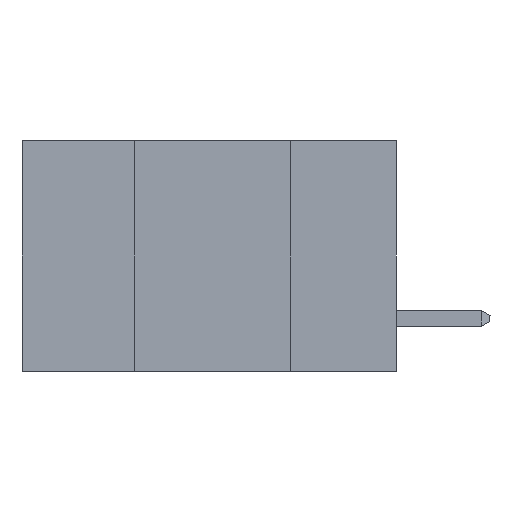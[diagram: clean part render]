
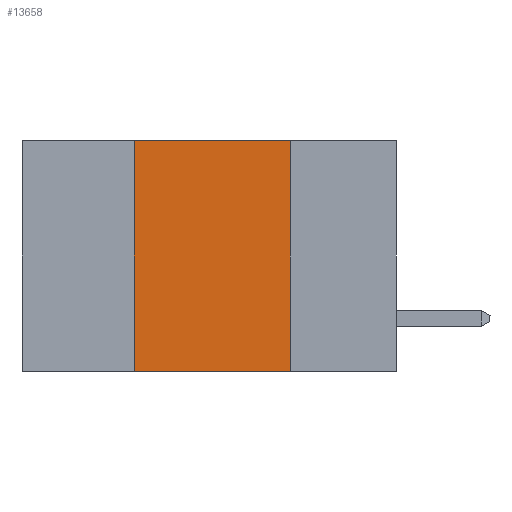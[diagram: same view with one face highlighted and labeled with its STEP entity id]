
A CAD part, left-side view. The second image highlights one B-rep face of the part: STEP entity #13658.
In plain terms, the highlighted planar face has unit normal (-1, 0, 0).
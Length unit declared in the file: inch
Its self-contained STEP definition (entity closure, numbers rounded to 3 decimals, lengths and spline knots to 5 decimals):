
#482 = EDGE_CURVE ( 'NONE', #15185, #2514, #15373, .T. ) ;
#598 = VERTEX_POINT ( 'NONE', #4691 ) ;
#778 = CARTESIAN_POINT ( 'NONE',  ( 0., 0.42, -0.37 ) ) ;
#888 = CARTESIAN_POINT ( 'NONE',  ( 0., 0.6, 0. ) ) ;
#2514 = VERTEX_POINT ( 'NONE', #10790 ) ;
#3417 = EDGE_LOOP ( 'NONE', ( #11002, #4985, #3614, #9863 ) ) ;
#3520 = DIRECTION ( 'NONE',  ( 0., 0., -1. ) ) ;
#3614 = ORIENTED_EDGE ( 'NONE', *, *, #12351, .F. ) ;
#3699 = VECTOR ( 'NONE', #4540, 39.37008 ) ;
#3708 = LINE ( 'NONE', #6241, #10955 ) ;
#3782 = DIRECTION ( 'NONE',  ( 0., 0., -1. ) ) ;
#4019 = VERTEX_POINT ( 'NONE', #778 ) ;
#4316 = LINE ( 'NONE', #14029, #6190 ) ;
#4540 = DIRECTION ( 'NONE',  ( 0., -1., 0. ) ) ;
#4691 = CARTESIAN_POINT ( 'NONE',  ( 0., 0.17, -0.37 ) ) ;
#4985 = ORIENTED_EDGE ( 'NONE', *, *, #482, .F. ) ;
#6190 = VECTOR ( 'NONE', #7683, 39.37008 ) ;
#6241 = CARTESIAN_POINT ( 'NONE',  ( 0., 0.17, -0.37 ) ) ;
#7103 = DIRECTION ( 'NONE',  ( 1., 0., 0. ) ) ;
#7683 = DIRECTION ( 'NONE',  ( 0., 0., 1. ) ) ;
#7903 = CARTESIAN_POINT ( 'NONE',  ( 0., 0.42, 0. ) ) ;
#8383 = CARTESIAN_POINT ( 'NONE',  ( 0., 0.6, 0. ) ) ;
#9418 = LINE ( 'NONE', #14105, #11992 ) ;
#9583 = FACE_OUTER_BOUND ( 'NONE', #3417, .T. ) ;
#9863 = ORIENTED_EDGE ( 'NONE', *, *, #13579, .T. ) ;
#10790 = CARTESIAN_POINT ( 'NONE',  ( 0., 0.17, 0. ) ) ;
#10955 = VECTOR ( 'NONE', #3782, 39.37008 ) ;
#11002 = ORIENTED_EDGE ( 'NONE', *, *, #14636, .F. ) ;
#11992 = VECTOR ( 'NONE', #14183, 39.37008 ) ;
#12351 = EDGE_CURVE ( 'NONE', #4019, #15185, #4316, .T. ) ;
#13579 = EDGE_CURVE ( 'NONE', #4019, #598, #9418, .T. ) ;
#13658 = ADVANCED_FACE ( 'NONE', ( #9583 ), #14642, .F. ) ;
#14029 = CARTESIAN_POINT ( 'NONE',  ( 0., 0.42, -0.37 ) ) ;
#14105 = CARTESIAN_POINT ( 'NONE',  ( 0., 0.6, -0.37 ) ) ;
#14183 = DIRECTION ( 'NONE',  ( 0., -1., 0. ) ) ;
#14636 = EDGE_CURVE ( 'NONE', #2514, #598, #3708, .T. ) ;
#14642 = PLANE ( 'NONE',  #15051 ) ;
#15051 = AXIS2_PLACEMENT_3D ( 'NONE', #8383, #7103, #3520 ) ;
#15185 = VERTEX_POINT ( 'NONE', #7903 ) ;
#15373 = LINE ( 'NONE', #888, #3699 ) ;
